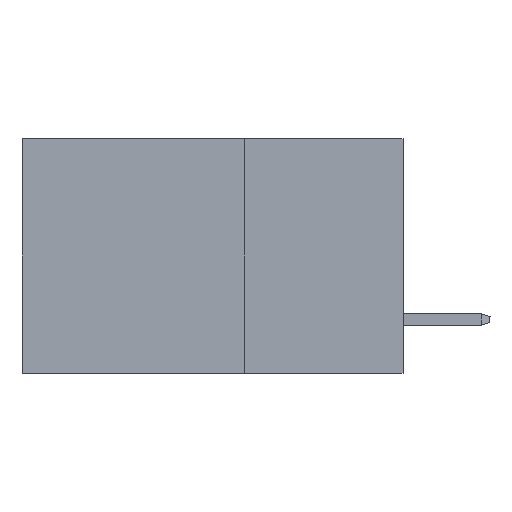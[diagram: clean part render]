
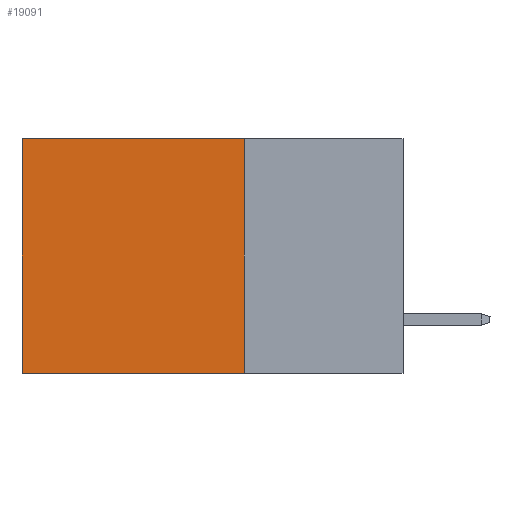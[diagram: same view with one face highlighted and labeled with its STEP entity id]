
A CAD part, left-side view. The second image highlights one B-rep face of the part: STEP entity #19091.
In plain terms, the highlighted planar face has unit normal (-1, 0, 0).
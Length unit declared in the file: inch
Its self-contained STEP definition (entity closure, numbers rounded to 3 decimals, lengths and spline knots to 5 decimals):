
#1379 = LINE ( 'NONE', #20846, #26037 ) ;
#1501 = DIRECTION ( 'NONE',  ( 0., 0., -1. ) ) ;
#1504 = ORIENTED_EDGE ( 'NONE', *, *, #25487, .F. ) ;
#1761 = VERTEX_POINT ( 'NONE', #25258 ) ;
#2132 = CARTESIAN_POINT ( 'NONE',  ( 0.2875, 0.25, -0.37 ) ) ;
#2692 = EDGE_CURVE ( 'NONE', #4543, #6914, #8131, .T. ) ;
#2769 = LINE ( 'NONE', #24096, #4625 ) ;
#3242 = VECTOR ( 'NONE', #5278, 39.37008 ) ;
#4134 = AXIS2_PLACEMENT_3D ( 'NONE', #25200, #18847, #1501 ) ;
#4543 = VERTEX_POINT ( 'NONE', #23594 ) ;
#4625 = VECTOR ( 'NONE', #9246, 39.37008 ) ;
#5278 = DIRECTION ( 'NONE',  ( 0., 0., -1. ) ) ;
#5331 = DIRECTION ( 'NONE',  ( 0., 0., -1. ) ) ;
#6119 = PLANE ( 'NONE',  #4134 ) ;
#6914 = VERTEX_POINT ( 'NONE', #20911 ) ;
#8131 = LINE ( 'NONE', #18329, #12388 ) ;
#8188 = ORIENTED_EDGE ( 'NONE', *, *, #13090, .T. ) ;
#8242 = FACE_OUTER_BOUND ( 'NONE', #21406, .T. ) ;
#9246 = DIRECTION ( 'NONE',  ( 0., 1., 0. ) ) ;
#11166 = VERTEX_POINT ( 'NONE', #2132 ) ;
#11494 = LINE ( 'NONE', #20374, #3242 ) ;
#12388 = VECTOR ( 'NONE', #5331, 39.37008 ) ;
#13090 = EDGE_CURVE ( 'NONE', #1761, #4543, #2769, .T. ) ;
#18329 = CARTESIAN_POINT ( 'NONE',  ( 0.2875, 0.6, 0. ) ) ;
#18740 = DIRECTION ( 'NONE',  ( 0., 1., 0. ) ) ;
#18847 = DIRECTION ( 'NONE',  ( 1., 0., 0. ) ) ;
#18987 = ORIENTED_EDGE ( 'NONE', *, *, #22470, .F. ) ;
#19091 = ADVANCED_FACE ( 'NONE', ( #8242 ), #6119, .F. ) ;
#20374 = CARTESIAN_POINT ( 'NONE',  ( 0.2875, 0.25, 0. ) ) ;
#20846 = CARTESIAN_POINT ( 'NONE',  ( 0.2875, 0.25, -0.37 ) ) ;
#20911 = CARTESIAN_POINT ( 'NONE',  ( 0.2875, 0.6, -0.37 ) ) ;
#21243 = ORIENTED_EDGE ( 'NONE', *, *, #2692, .T. ) ;
#21406 = EDGE_LOOP ( 'NONE', ( #21243, #1504, #18987, #8188 ) ) ;
#22470 = EDGE_CURVE ( 'NONE', #1761, #11166, #11494, .T. ) ;
#23594 = CARTESIAN_POINT ( 'NONE',  ( 0.2875, 0.6, 0. ) ) ;
#24096 = CARTESIAN_POINT ( 'NONE',  ( 0.2875, 0.25, 0. ) ) ;
#25200 = CARTESIAN_POINT ( 'NONE',  ( 0.2875, 0.25, 0. ) ) ;
#25258 = CARTESIAN_POINT ( 'NONE',  ( 0.2875, 0.25, 0. ) ) ;
#25487 = EDGE_CURVE ( 'NONE', #11166, #6914, #1379, .T. ) ;
#26037 = VECTOR ( 'NONE', #18740, 39.37008 ) ;
